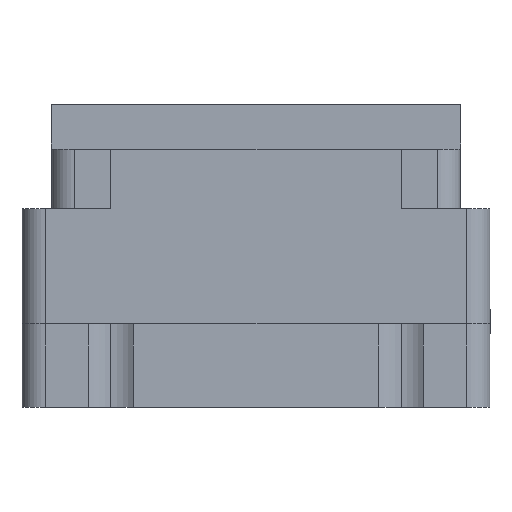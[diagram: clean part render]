
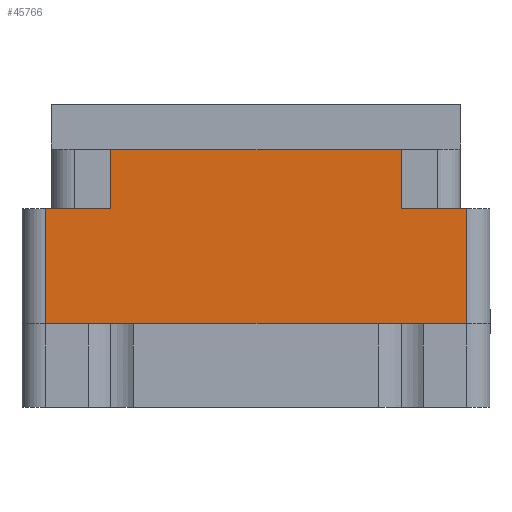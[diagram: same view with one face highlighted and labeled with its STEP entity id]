
A CAD part, left-side view. The second image highlights one B-rep face of the part: STEP entity #45766.
In plain terms, the highlighted planar face has unit normal (-1, 0, 0).
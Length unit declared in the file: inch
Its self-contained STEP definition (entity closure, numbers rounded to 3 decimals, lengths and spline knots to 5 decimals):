
#121 = CARTESIAN_POINT ( 'NONE',  ( -1.359, -0.3825, -0.274 ) ) ;
#946 = EDGE_CURVE ( 'NONE', #37624, #3914, #43759, .T. ) ;
#2332 = VERTEX_POINT ( 'NONE', #52153 ) ;
#3046 = LINE ( 'NONE', #58875, #60274 ) ;
#3914 = VERTEX_POINT ( 'NONE', #43746 ) ;
#4876 = LINE ( 'NONE', #17134, #24518 ) ;
#7255 = LINE ( 'NONE', #49543, #62208 ) ;
#7966 = DIRECTION ( 'NONE',  ( 0., 0., 1. ) ) ;
#8165 = CARTESIAN_POINT ( 'NONE',  ( -1.359, -0.617, -0.798 ) ) ;
#9900 = DIRECTION ( 'NONE',  ( 0., 0., -1. ) ) ;
#10357 = ORIENTED_EDGE ( 'NONE', *, *, #42540, .T. ) ;
#11036 = CARTESIAN_POINT ( 'NONE',  ( -1.359, 0., -0.578 ) ) ;
#11585 = VERTEX_POINT ( 'NONE', #36504 ) ;
#12297 = DIRECTION ( 'NONE',  ( 0., -1., 0. ) ) ;
#12866 = CARTESIAN_POINT ( 'NONE',  ( -1.359, -0.3825, -0.274 ) ) ;
#13656 = LINE ( 'NONE', #45159, #21229 ) ;
#13809 = AXIS2_PLACEMENT_3D ( 'NONE', #8165, #33062, #7966 ) ;
#14692 = ORIENTED_EDGE ( 'NONE', *, *, #48684, .T. ) ;
#16102 = DIRECTION ( 'NONE',  ( 0., -1., 0. ) ) ;
#16144 = ORIENTED_EDGE ( 'NONE', *, *, #57423, .T. ) ;
#17134 = CARTESIAN_POINT ( 'NONE',  ( -1.359, 0., -0.274 ) ) ;
#18375 = VECTOR ( 'NONE', #26227, 39.37008 ) ;
#21229 = VECTOR ( 'NONE', #12297, 39.37008 ) ;
#21382 = VECTOR ( 'NONE', #57152, 39.37008 ) ;
#22529 = CARTESIAN_POINT ( 'NONE',  ( -1.359, 0.555, -0.274 ) ) ;
#24518 = VECTOR ( 'NONE', #60391, 39.37008 ) ;
#24781 = EDGE_CURVE ( 'NONE', #11585, #25376, #13656, .T. ) ;
#25236 = DIRECTION ( 'NONE',  ( 0., 0., 1. ) ) ;
#25376 = VERTEX_POINT ( 'NONE', #53372 ) ;
#25536 = DIRECTION ( 'NONE',  ( 0., 0., 1. ) ) ;
#25876 = LINE ( 'NONE', #121, #21382 ) ;
#26227 = DIRECTION ( 'NONE',  ( 0., -1., 0. ) ) ;
#28273 = ORIENTED_EDGE ( 'NONE', *, *, #48865, .T. ) ;
#28769 = CARTESIAN_POINT ( 'NONE',  ( -1.359, -0.555, -0.578 ) ) ;
#31153 = LINE ( 'NONE', #11036, #18375 ) ;
#33062 = DIRECTION ( 'NONE',  ( -1., 0., 0. ) ) ;
#35436 = LINE ( 'NONE', #52653, #60227 ) ;
#35584 = EDGE_CURVE ( 'NONE', #3914, #11585, #7255, .T. ) ;
#36504 = CARTESIAN_POINT ( 'NONE',  ( -1.359, 0.3825, -0.117 ) ) ;
#37095 = PLANE ( 'NONE',  #13809 ) ;
#37394 = ORIENTED_EDGE ( 'NONE', *, *, #946, .F. ) ;
#37624 = VERTEX_POINT ( 'NONE', #22529 ) ;
#38593 = CARTESIAN_POINT ( 'NONE',  ( -1.359, -0.555, -0.274 ) ) ;
#40116 = CARTESIAN_POINT ( 'NONE',  ( -1.359, 0., -0.274 ) ) ;
#40483 = EDGE_LOOP ( 'NONE', ( #37394, #16144, #28273, #10357, #42510, #14692, #43040, #60446 ) ) ;
#42510 = ORIENTED_EDGE ( 'NONE', *, *, #47559, .F. ) ;
#42540 = EDGE_CURVE ( 'NONE', #49523, #54132, #3046, .T. ) ;
#43040 = ORIENTED_EDGE ( 'NONE', *, *, #24781, .F. ) ;
#43746 = CARTESIAN_POINT ( 'NONE',  ( -1.359, 0.3825, -0.274 ) ) ;
#43759 = LINE ( 'NONE', #40116, #51342 ) ;
#45159 = CARTESIAN_POINT ( 'NONE',  ( -1.359, 0.617, -0.117 ) ) ;
#45766 = ADVANCED_FACE ( 'NONE', ( #52639 ), #37095, .T. ) ;
#47559 = EDGE_CURVE ( 'NONE', #60645, #54132, #4876, .T. ) ;
#48684 = EDGE_CURVE ( 'NONE', #60645, #25376, #25876, .T. ) ;
#48865 = EDGE_CURVE ( 'NONE', #2332, #49523, #31153, .T. ) ;
#49523 = VERTEX_POINT ( 'NONE', #28769 ) ;
#49543 = CARTESIAN_POINT ( 'NONE',  ( -1.359, 0.3825, -0.274 ) ) ;
#51342 = VECTOR ( 'NONE', #16102, 39.37008 ) ;
#52153 = CARTESIAN_POINT ( 'NONE',  ( -1.359, 0.555, -0.578 ) ) ;
#52639 = FACE_OUTER_BOUND ( 'NONE', #40483, .T. ) ;
#52653 = CARTESIAN_POINT ( 'NONE',  ( -1.359, 0.555, -0.798 ) ) ;
#53372 = CARTESIAN_POINT ( 'NONE',  ( -1.359, -0.3825, -0.117 ) ) ;
#54132 = VERTEX_POINT ( 'NONE', #38593 ) ;
#57152 = DIRECTION ( 'NONE',  ( 0., 0., 1. ) ) ;
#57423 = EDGE_CURVE ( 'NONE', #37624, #2332, #35436, .T. ) ;
#58875 = CARTESIAN_POINT ( 'NONE',  ( -1.359, -0.555, -0.798 ) ) ;
#60227 = VECTOR ( 'NONE', #9900, 39.37008 ) ;
#60274 = VECTOR ( 'NONE', #25236, 39.37008 ) ;
#60391 = DIRECTION ( 'NONE',  ( 0., -1., 0. ) ) ;
#60446 = ORIENTED_EDGE ( 'NONE', *, *, #35584, .F. ) ;
#60645 = VERTEX_POINT ( 'NONE', #12866 ) ;
#62208 = VECTOR ( 'NONE', #25536, 39.37008 ) ;
